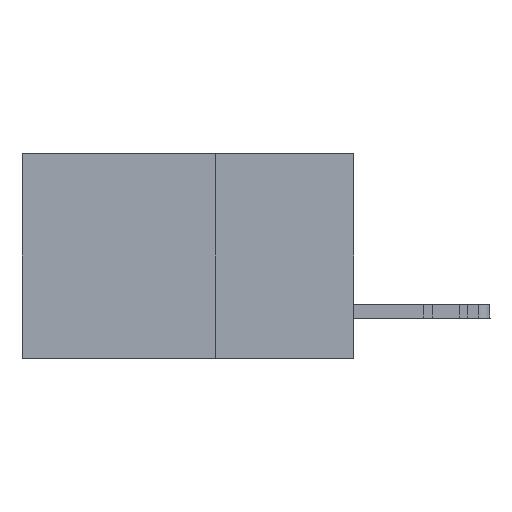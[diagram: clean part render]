
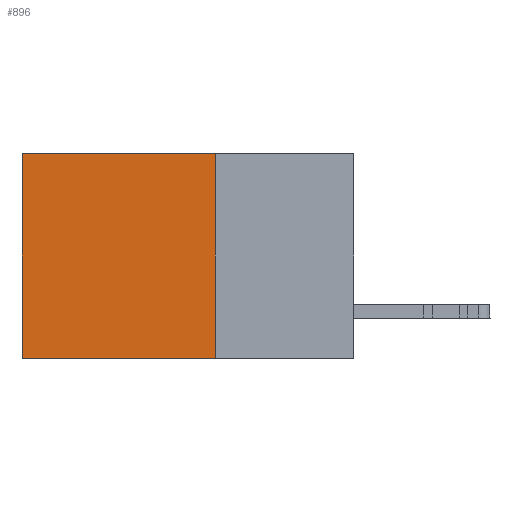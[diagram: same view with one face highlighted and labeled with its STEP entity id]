
A CAD part, left-side view. The second image highlights one B-rep face of the part: STEP entity #896.
In plain terms, the highlighted planar face has unit normal (-1, 0, 0).
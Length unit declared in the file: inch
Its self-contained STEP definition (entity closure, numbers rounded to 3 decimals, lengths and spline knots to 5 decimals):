
#896 = ADVANCED_FACE ( 'NONE', ( #14836 ), #1331, .F. ) ;
#1331 = PLANE ( 'NONE',  #11685 ) ;
#2890 = EDGE_CURVE ( 'NONE', #27728, #23241, #29460, .T. ) ;
#3199 = CARTESIAN_POINT ( 'NONE',  ( 0.2875, 0.25, -0.37 ) ) ;
#5982 = VERTEX_POINT ( 'NONE', #20701 ) ;
#7975 = LINE ( 'NONE', #13950, #14853 ) ;
#9676 = CARTESIAN_POINT ( 'NONE',  ( 0.2875, 0.6, 0. ) ) ;
#10657 = DIRECTION ( 'NONE',  ( 0., 1., 0. ) ) ;
#11272 = LINE ( 'NONE', #9676, #30896 ) ;
#11685 = AXIS2_PLACEMENT_3D ( 'NONE', #21588, #34706, #34858 ) ;
#12037 = CARTESIAN_POINT ( 'NONE',  ( 0.2875, 0.25, -0.37 ) ) ;
#13950 = CARTESIAN_POINT ( 'NONE',  ( 0.2875, 0.25, 0. ) ) ;
#14576 = LINE ( 'NONE', #34755, #36226 ) ;
#14836 = FACE_OUTER_BOUND ( 'NONE', #23913, .T. ) ;
#14853 = VECTOR ( 'NONE', #34614, 39.37008 ) ;
#16264 = ORIENTED_EDGE ( 'NONE', *, *, #26420, .T. ) ;
#16632 = DIRECTION ( 'NONE',  ( 0., 0., -1. ) ) ;
#16995 = EDGE_CURVE ( 'NONE', #23647, #23241, #11272, .T. ) ;
#19829 = CARTESIAN_POINT ( 'NONE',  ( 0.2875, 0.6, 0. ) ) ;
#20701 = CARTESIAN_POINT ( 'NONE',  ( 0.2875, 0.25, 0. ) ) ;
#21588 = CARTESIAN_POINT ( 'NONE',  ( 0.2875, 0.25, 0. ) ) ;
#23107 = ORIENTED_EDGE ( 'NONE', *, *, #16995, .T. ) ;
#23241 = VERTEX_POINT ( 'NONE', #30182 ) ;
#23647 = VERTEX_POINT ( 'NONE', #19829 ) ;
#23913 = EDGE_LOOP ( 'NONE', ( #23107, #36089, #38272, #16264 ) ) ;
#26420 = EDGE_CURVE ( 'NONE', #5982, #23647, #14576, .T. ) ;
#27728 = VERTEX_POINT ( 'NONE', #3199 ) ;
#28503 = DIRECTION ( 'NONE',  ( 0., 1., 0. ) ) ;
#29460 = LINE ( 'NONE', #12037, #42156 ) ;
#30182 = CARTESIAN_POINT ( 'NONE',  ( 0.2875, 0.6, -0.37 ) ) ;
#30896 = VECTOR ( 'NONE', #16632, 39.37008 ) ;
#34614 = DIRECTION ( 'NONE',  ( 0., 0., -1. ) ) ;
#34706 = DIRECTION ( 'NONE',  ( 1., 0., 0. ) ) ;
#34755 = CARTESIAN_POINT ( 'NONE',  ( 0.2875, 0.25, 0. ) ) ;
#34858 = DIRECTION ( 'NONE',  ( 0., 0., -1. ) ) ;
#36089 = ORIENTED_EDGE ( 'NONE', *, *, #2890, .F. ) ;
#36112 = EDGE_CURVE ( 'NONE', #5982, #27728, #7975, .T. ) ;
#36226 = VECTOR ( 'NONE', #10657, 39.37008 ) ;
#38272 = ORIENTED_EDGE ( 'NONE', *, *, #36112, .F. ) ;
#42156 = VECTOR ( 'NONE', #28503, 39.37008 ) ;
